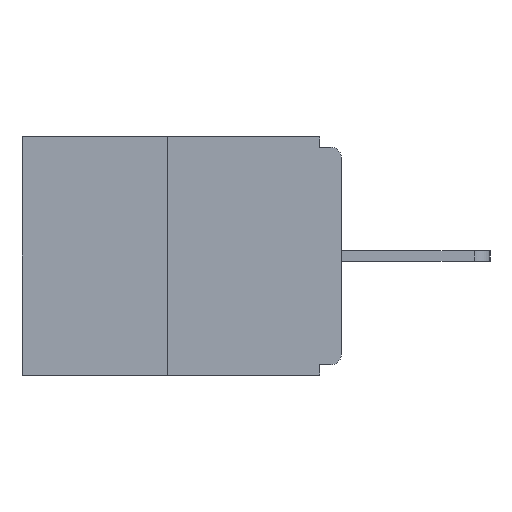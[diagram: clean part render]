
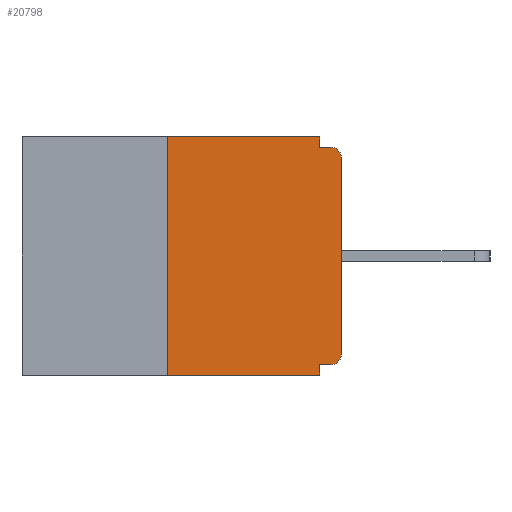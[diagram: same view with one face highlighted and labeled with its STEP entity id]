
A CAD part, left-side view. The second image highlights one B-rep face of the part: STEP entity #20798.
In plain terms, the highlighted planar face has unit normal (-1, 0, 0).
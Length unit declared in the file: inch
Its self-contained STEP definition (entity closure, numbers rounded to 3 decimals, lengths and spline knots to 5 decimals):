
#58 = DIRECTION ( 'NONE',  ( 0., 0., 1. ) ) ;
#94 = CIRCLE ( 'NONE', #20008, 0.015 ) ;
#258 = EDGE_CURVE ( 'NONE', #18923, #3006, #16711, .T. ) ;
#620 = EDGE_CURVE ( 'NONE', #1743, #11910, #14018, .T. ) ;
#1037 = CARTESIAN_POINT ( 'NONE',  ( 0., 0.25, -0.343 ) ) ;
#1294 = CARTESIAN_POINT ( 'NONE',  ( 0., 0.031, -0.343 ) ) ;
#1743 = VERTEX_POINT ( 'NONE', #7206 ) ;
#1770 = EDGE_CURVE ( 'NONE', #18094, #18923, #13639, .T. ) ;
#2194 = DIRECTION ( 'NONE',  ( 0., 1., 0. ) ) ;
#2511 = VERTEX_POINT ( 'NONE', #8477 ) ;
#2680 = DIRECTION ( 'NONE',  ( 1., 0., 0. ) ) ;
#2709 = VECTOR ( 'NONE', #17513, 39.37008 ) ;
#2904 = CIRCLE ( 'NONE', #7577, 0.015 ) ;
#3006 = VERTEX_POINT ( 'NONE', #8142 ) ;
#3062 = EDGE_CURVE ( 'NONE', #11910, #10019, #5781, .T. ) ;
#3255 = ORIENTED_EDGE ( 'NONE', *, *, #258, .F. ) ;
#3277 = DIRECTION ( 'NONE',  ( 0., 0., -1. ) ) ;
#3631 = VECTOR ( 'NONE', #58, 39.37008 ) ;
#3678 = CARTESIAN_POINT ( 'NONE',  ( 0., 0.25, 0. ) ) ;
#3762 = CARTESIAN_POINT ( 'NONE',  ( 0., 0., -0.313 ) ) ;
#3975 = CARTESIAN_POINT ( 'NONE',  ( 0., 0.031, 0. ) ) ;
#4217 = LINE ( 'NONE', #10266, #3631 ) ;
#4218 = VERTEX_POINT ( 'NONE', #4755 ) ;
#4317 = EDGE_CURVE ( 'NONE', #20972, #10019, #13205, .T. ) ;
#4755 = CARTESIAN_POINT ( 'NONE',  ( 0., 0.015, -0.015 ) ) ;
#5599 = EDGE_CURVE ( 'NONE', #20972, #18094, #19956, .T. ) ;
#5717 = VECTOR ( 'NONE', #14176, 39.37008 ) ;
#5781 = LINE ( 'NONE', #1294, #14416 ) ;
#5914 = EDGE_CURVE ( 'NONE', #22073, #2511, #4217, .T. ) ;
#7095 = DIRECTION ( 'NONE',  ( 0., 0., -1. ) ) ;
#7206 = CARTESIAN_POINT ( 'NONE',  ( 0., 0.015, -0.328 ) ) ;
#7577 = AXIS2_PLACEMENT_3D ( 'NONE', #19770, #9266, #21483 ) ;
#8099 = EDGE_LOOP ( 'NONE', ( #14484, #15345, #17207, #16341, #12643, #11028, #13015, #10448, #10808, #3255 ) ) ;
#8113 = CARTESIAN_POINT ( 'NONE',  ( 0., 0.46, 0. ) ) ;
#8142 = CARTESIAN_POINT ( 'NONE',  ( 0., 0.031, -0.015 ) ) ;
#8477 = CARTESIAN_POINT ( 'NONE',  ( 0., 0., -0.03 ) ) ;
#8741 = DIRECTION ( 'NONE',  ( 0., -1., 0. ) ) ;
#9266 = DIRECTION ( 'NONE',  ( -1., 0., 0. ) ) ;
#9539 = AXIS2_PLACEMENT_3D ( 'NONE', #13829, #2680, #15581 ) ;
#9816 = VECTOR ( 'NONE', #17551, 39.37008 ) ;
#10019 = VERTEX_POINT ( 'NONE', #16274 ) ;
#10266 = CARTESIAN_POINT ( 'NONE',  ( 0., 0., 0. ) ) ;
#10377 = LINE ( 'NONE', #15769, #9816 ) ;
#10448 = ORIENTED_EDGE ( 'NONE', *, *, #13786, .T. ) ;
#10519 = CARTESIAN_POINT ( 'NONE',  ( 0., 0.031, -0.328 ) ) ;
#10587 = DIRECTION ( 'NONE',  ( -1., 0., 0. ) ) ;
#10808 = ORIENTED_EDGE ( 'NONE', *, *, #19541, .F. ) ;
#11028 = ORIENTED_EDGE ( 'NONE', *, *, #17320, .T. ) ;
#11910 = VERTEX_POINT ( 'NONE', #10519 ) ;
#11996 = VECTOR ( 'NONE', #3277, 39.37008 ) ;
#12643 = ORIENTED_EDGE ( 'NONE', *, *, #620, .F. ) ;
#13015 = ORIENTED_EDGE ( 'NONE', *, *, #5914, .T. ) ;
#13205 = LINE ( 'NONE', #21890, #2709 ) ;
#13639 = LINE ( 'NONE', #8113, #17748 ) ;
#13786 = EDGE_CURVE ( 'NONE', #2511, #4218, #94, .T. ) ;
#13829 = CARTESIAN_POINT ( 'NONE',  ( 0., 0.46, 0. ) ) ;
#14018 = LINE ( 'NONE', #22154, #18112 ) ;
#14176 = DIRECTION ( 'NONE',  ( 0., 0., 1. ) ) ;
#14416 = VECTOR ( 'NONE', #7095, 39.37008 ) ;
#14484 = ORIENTED_EDGE ( 'NONE', *, *, #1770, .F. ) ;
#15345 = ORIENTED_EDGE ( 'NONE', *, *, #5599, .F. ) ;
#15581 = DIRECTION ( 'NONE',  ( 0., 0., -1. ) ) ;
#15769 = CARTESIAN_POINT ( 'NONE',  ( 0., 0., -0.015 ) ) ;
#15906 = FACE_OUTER_BOUND ( 'NONE', #8099, .T. ) ;
#16274 = CARTESIAN_POINT ( 'NONE',  ( 0., 0.031, -0.343 ) ) ;
#16341 = ORIENTED_EDGE ( 'NONE', *, *, #3062, .F. ) ;
#16497 = CARTESIAN_POINT ( 'NONE',  ( 0., 0.25, 0. ) ) ;
#16711 = LINE ( 'NONE', #3975, #11996 ) ;
#17207 = ORIENTED_EDGE ( 'NONE', *, *, #4317, .T. ) ;
#17295 = PLANE ( 'NONE',  #9539 ) ;
#17320 = EDGE_CURVE ( 'NONE', #1743, #22073, #2904, .T. ) ;
#17513 = DIRECTION ( 'NONE',  ( 0., -1., 0. ) ) ;
#17551 = DIRECTION ( 'NONE',  ( 0., -1., 0. ) ) ;
#17724 = CARTESIAN_POINT ( 'NONE',  ( 0., 0.031, 0. ) ) ;
#17748 = VECTOR ( 'NONE', #8741, 39.37008 ) ;
#18094 = VERTEX_POINT ( 'NONE', #16497 ) ;
#18112 = VECTOR ( 'NONE', #2194, 39.37008 ) ;
#18923 = VERTEX_POINT ( 'NONE', #17724 ) ;
#19541 = EDGE_CURVE ( 'NONE', #3006, #4218, #10377, .T. ) ;
#19770 = CARTESIAN_POINT ( 'NONE',  ( 0., 0.015, -0.313 ) ) ;
#19956 = LINE ( 'NONE', #3678, #5717 ) ;
#20008 = AXIS2_PLACEMENT_3D ( 'NONE', #21026, #10587, #22688 ) ;
#20798 = ADVANCED_FACE ( 'NONE', ( #15906 ), #17295, .F. ) ;
#20972 = VERTEX_POINT ( 'NONE', #1037 ) ;
#21026 = CARTESIAN_POINT ( 'NONE',  ( 0., 0.015, -0.03 ) ) ;
#21483 = DIRECTION ( 'NONE',  ( 0., 0., -1. ) ) ;
#21890 = CARTESIAN_POINT ( 'NONE',  ( 0., 0.46, -0.343 ) ) ;
#22073 = VERTEX_POINT ( 'NONE', #3762 ) ;
#22154 = CARTESIAN_POINT ( 'NONE',  ( 0., 0., -0.328 ) ) ;
#22688 = DIRECTION ( 'NONE',  ( 0., 0., -1. ) ) ;
